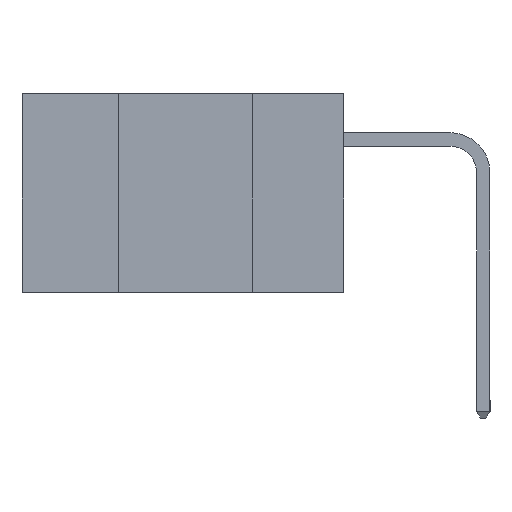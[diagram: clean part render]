
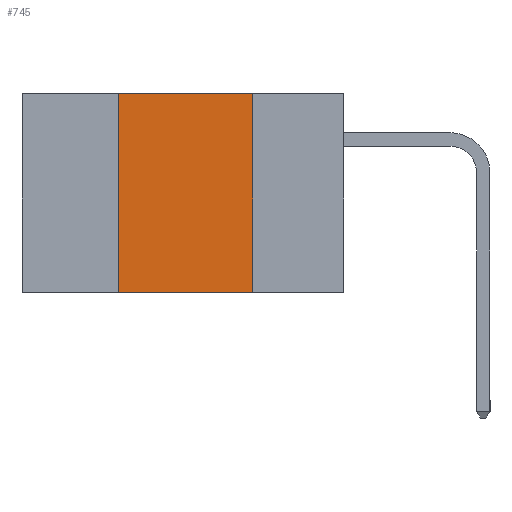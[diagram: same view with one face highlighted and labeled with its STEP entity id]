
A CAD part, left-side view. The second image highlights one B-rep face of the part: STEP entity #745.
In plain terms, the highlighted planar face has unit normal (-1, 0, 0).
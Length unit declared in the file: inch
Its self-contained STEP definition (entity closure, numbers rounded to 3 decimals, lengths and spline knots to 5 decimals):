
#376 = VERTEX_POINT ( 'NONE', #16584 ) ;
#745 = ADVANCED_FACE ( 'NONE', ( #5655 ), #9573, .F. ) ;
#842 = EDGE_CURVE ( 'NONE', #20902, #376, #19820, .T. ) ;
#1388 = AXIS2_PLACEMENT_3D ( 'NONE', #15188, #15394, #19536 ) ;
#1977 = DIRECTION ( 'NONE',  ( 0., 0., -1. ) ) ;
#2608 = VECTOR ( 'NONE', #22124, 39.37008 ) ;
#2698 = CARTESIAN_POINT ( 'NONE',  ( 0., 0.17, -0.37 ) ) ;
#2743 = EDGE_CURVE ( 'NONE', #23241, #20902, #4903, .T. ) ;
#3801 = CARTESIAN_POINT ( 'NONE',  ( 0., 0.42, 0. ) ) ;
#4834 = VERTEX_POINT ( 'NONE', #18920 ) ;
#4903 = LINE ( 'NONE', #11997, #12167 ) ;
#5655 = FACE_OUTER_BOUND ( 'NONE', #19334, .T. ) ;
#6145 = CARTESIAN_POINT ( 'NONE',  ( 0., 0.42, -0.37 ) ) ;
#8551 = VECTOR ( 'NONE', #1977, 39.37008 ) ;
#8689 = LINE ( 'NONE', #6145, #2608 ) ;
#9573 = PLANE ( 'NONE',  #1388 ) ;
#10705 = ORIENTED_EDGE ( 'NONE', *, *, #24478, .T. ) ;
#11755 = DIRECTION ( 'NONE',  ( 0., -1., 0. ) ) ;
#11997 = CARTESIAN_POINT ( 'NONE',  ( 0., 0.6, 0. ) ) ;
#12167 = VECTOR ( 'NONE', #11755, 39.37008 ) ;
#15188 = CARTESIAN_POINT ( 'NONE',  ( 0., 0.6, 0. ) ) ;
#15394 = DIRECTION ( 'NONE',  ( 1., 0., 0. ) ) ;
#15495 = CARTESIAN_POINT ( 'NONE',  ( 0., 0.17, 0. ) ) ;
#16584 = CARTESIAN_POINT ( 'NONE',  ( 0., 0.17, -0.37 ) ) ;
#18884 = ORIENTED_EDGE ( 'NONE', *, *, #2743, .F. ) ;
#18920 = CARTESIAN_POINT ( 'NONE',  ( 0., 0.42, -0.37 ) ) ;
#19064 = VECTOR ( 'NONE', #20108, 39.37008 ) ;
#19334 = EDGE_LOOP ( 'NONE', ( #21621, #18884, #25226, #10705 ) ) ;
#19536 = DIRECTION ( 'NONE',  ( 0., 0., -1. ) ) ;
#19820 = LINE ( 'NONE', #2698, #8551 ) ;
#20108 = DIRECTION ( 'NONE',  ( 0., -1., 0. ) ) ;
#20902 = VERTEX_POINT ( 'NONE', #15495 ) ;
#21621 = ORIENTED_EDGE ( 'NONE', *, *, #842, .F. ) ;
#22124 = DIRECTION ( 'NONE',  ( 0., 0., 1. ) ) ;
#22705 = EDGE_CURVE ( 'NONE', #4834, #23241, #8689, .T. ) ;
#23241 = VERTEX_POINT ( 'NONE', #3801 ) ;
#23883 = CARTESIAN_POINT ( 'NONE',  ( 0., 0.6, -0.37 ) ) ;
#24208 = LINE ( 'NONE', #23883, #19064 ) ;
#24478 = EDGE_CURVE ( 'NONE', #4834, #376, #24208, .T. ) ;
#25226 = ORIENTED_EDGE ( 'NONE', *, *, #22705, .F. ) ;
